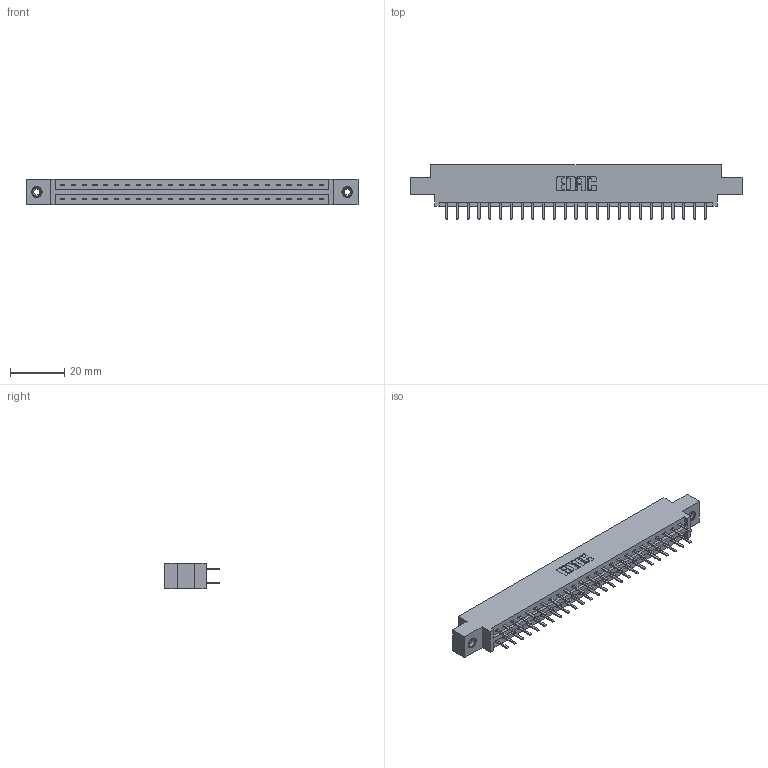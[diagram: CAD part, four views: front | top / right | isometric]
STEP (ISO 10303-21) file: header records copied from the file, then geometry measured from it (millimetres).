
FILE_DESCRIPTION (( 'STEP AP203' ), '1' );
FILE_NAME ('387-050-520-808.STEP', '2018-09-20T07:24:01', ( '' ), ( '' ), 'SwSTEP 2.0', 'SolidWorks 2016', '' );
FILE_SCHEMA (( 'CONFIG_CONTROL_DESIGN' ));
Length unit declared in the file: inch
Products named in the file (4): 337 Part_0.170 Offset - 0.156 Dia-TI; 345-292-001_345-293-120; 345-250-001_345-250-003-102; 387-050-520-808
Assembly tree (53 placements, depth 2):
  387-050-520-808
    337 Part_0.170 Offset - 0.156 Dia-TI
    345-292-001_345-293-120  x50
    345-250-001_345-250-003-102  x2
Bounding box: 122.07 x 20.02 x 9.4 mm (x, y, z)
Volume: 12492.7 mm3; surface area: 14026.9 mm2
Topology: 53 solids, 53 shells, 3078 faces, 8909 edges, 5798 vertices
Faces by surface type: plane 2106, cylinder 956, cone 12, torus 4
Entity records: 23014 total; most frequent: CARTESIAN_POINT 3885, ORIENTED_EDGE 3802, DIRECTION 3355, EDGE_CURVE 1901, LINE 1749, VECTOR 1749, VERTEX_POINT 1260, AXIS2_PLACEMENT_3D 803
